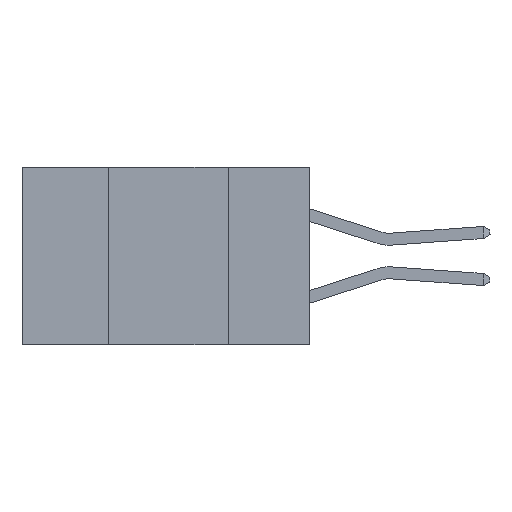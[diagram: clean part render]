
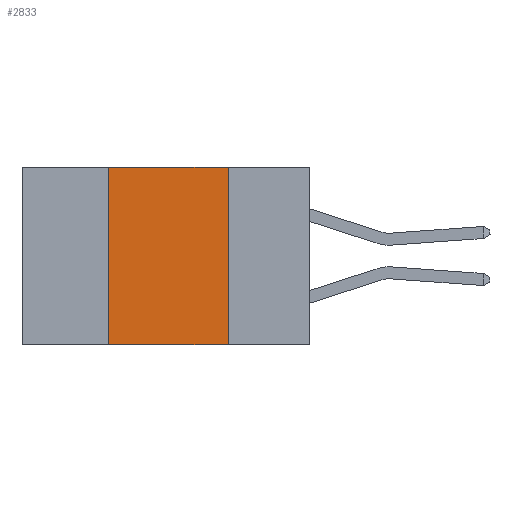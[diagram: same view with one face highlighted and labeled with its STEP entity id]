
A CAD part, left-side view. The second image highlights one B-rep face of the part: STEP entity #2833.
In plain terms, the highlighted planar face has unit normal (-1, 0, 0).
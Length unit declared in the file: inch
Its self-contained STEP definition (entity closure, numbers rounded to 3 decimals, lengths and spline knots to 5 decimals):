
#372 = CARTESIAN_POINT ( 'NONE',  ( 0., 0.42, 0. ) ) ;
#1136 = CARTESIAN_POINT ( 'NONE',  ( 0., 0.6, 0. ) ) ;
#1203 = DIRECTION ( 'NONE',  ( 0., -1., 0. ) ) ;
#1676 = FACE_OUTER_BOUND ( 'NONE', #6454, .T. ) ;
#2200 = CARTESIAN_POINT ( 'NONE',  ( 0., 0.17, 0. ) ) ;
#2502 = ORIENTED_EDGE ( 'NONE', *, *, #12794, .F. ) ;
#2763 = VECTOR ( 'NONE', #12365, 39.37008 ) ;
#2833 = ADVANCED_FACE ( 'NONE', ( #1676 ), #13162, .F. ) ;
#2965 = CARTESIAN_POINT ( 'NONE',  ( 0., 0.42, -0.37 ) ) ;
#3006 = DIRECTION ( 'NONE',  ( 0., 0., 1. ) ) ;
#4077 = ORIENTED_EDGE ( 'NONE', *, *, #4481, .F. ) ;
#4481 = EDGE_CURVE ( 'NONE', #5637, #12176, #8438, .T. ) ;
#4959 = VERTEX_POINT ( 'NONE', #8509 ) ;
#5637 = VERTEX_POINT ( 'NONE', #2200 ) ;
#6011 = EDGE_CURVE ( 'NONE', #13879, #5637, #7003, .T. ) ;
#6454 = EDGE_LOOP ( 'NONE', ( #4077, #10450, #2502, #8981 ) ) ;
#6633 = VECTOR ( 'NONE', #1203, 39.37008 ) ;
#6987 = CARTESIAN_POINT ( 'NONE',  ( 0., 0.6, -0.37 ) ) ;
#6988 = DIRECTION ( 'NONE',  ( 0., -1., 0. ) ) ;
#7003 = LINE ( 'NONE', #1136, #6633 ) ;
#7552 = VECTOR ( 'NONE', #6988, 39.37008 ) ;
#8186 = AXIS2_PLACEMENT_3D ( 'NONE', #8826, #11323, #11306 ) ;
#8438 = LINE ( 'NONE', #12509, #2763 ) ;
#8509 = CARTESIAN_POINT ( 'NONE',  ( 0., 0.42, -0.37 ) ) ;
#8826 = CARTESIAN_POINT ( 'NONE',  ( 0., 0.6, 0. ) ) ;
#8981 = ORIENTED_EDGE ( 'NONE', *, *, #9801, .T. ) ;
#9397 = CARTESIAN_POINT ( 'NONE',  ( 0., 0.17, -0.37 ) ) ;
#9801 = EDGE_CURVE ( 'NONE', #4959, #12176, #10558, .T. ) ;
#10450 = ORIENTED_EDGE ( 'NONE', *, *, #6011, .F. ) ;
#10558 = LINE ( 'NONE', #6987, #7552 ) ;
#10638 = LINE ( 'NONE', #2965, #12888 ) ;
#11306 = DIRECTION ( 'NONE',  ( 0., 0., -1. ) ) ;
#11323 = DIRECTION ( 'NONE',  ( 1., 0., 0. ) ) ;
#12176 = VERTEX_POINT ( 'NONE', #9397 ) ;
#12365 = DIRECTION ( 'NONE',  ( 0., 0., -1. ) ) ;
#12509 = CARTESIAN_POINT ( 'NONE',  ( 0., 0.17, -0.37 ) ) ;
#12794 = EDGE_CURVE ( 'NONE', #4959, #13879, #10638, .T. ) ;
#12888 = VECTOR ( 'NONE', #3006, 39.37008 ) ;
#13162 = PLANE ( 'NONE',  #8186 ) ;
#13879 = VERTEX_POINT ( 'NONE', #372 ) ;
